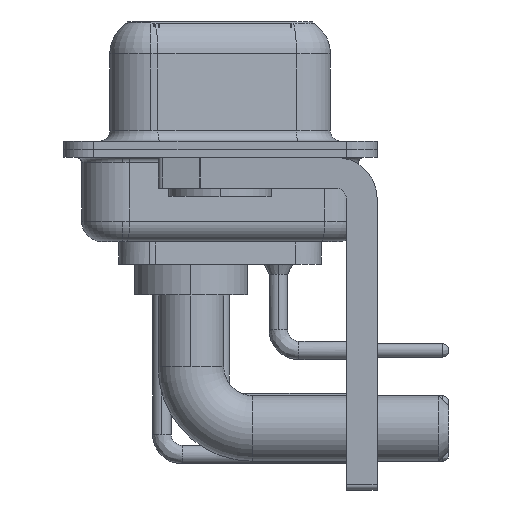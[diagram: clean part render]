
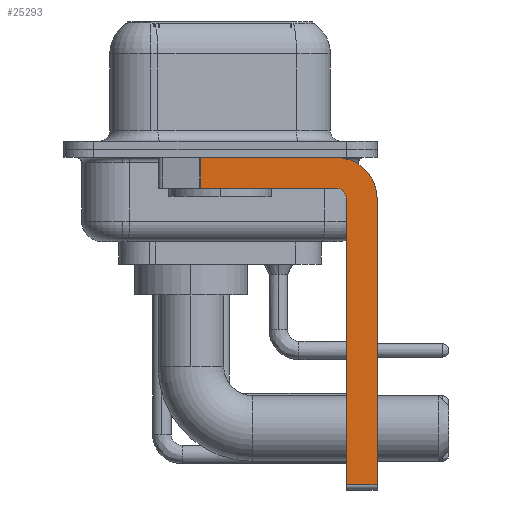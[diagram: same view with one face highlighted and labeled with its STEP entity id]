
A CAD part, left-side view. The second image highlights one B-rep face of the part: STEP entity #25293.
In plain terms, the highlighted planar face has unit normal (-1, 0, 0).
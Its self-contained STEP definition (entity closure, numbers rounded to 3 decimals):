
#324 = CARTESIAN_POINT ( 'NONE',  ( -2.9, -5.65, -16.35 ) ) ;
#525 = DIRECTION ( 'NONE',  ( 0., 0., 1. ) ) ;
#981 = CARTESIAN_POINT ( 'NONE',  ( -2.9, -7.65, -2.4 ) ) ;
#1199 = EDGE_CURVE ( 'NONE', #22641, #16061, #11977, .T. ) ;
#1399 = CIRCLE ( 'NONE', #16480, 0.5 ) ;
#1615 = CARTESIAN_POINT ( 'NONE',  ( -2.9, 0.978, -1.9 ) ) ;
#2493 = VERTEX_POINT ( 'NONE', #981 ) ;
#2877 = ORIENTED_EDGE ( 'NONE', *, *, #9466, .T. ) ;
#2976 = DIRECTION ( 'NONE',  ( 0., -1., 0. ) ) ;
#3555 = ORIENTED_EDGE ( 'NONE', *, *, #12667, .F. ) ;
#4824 = EDGE_CURVE ( 'NONE', #22641, #5567, #7491, .T. ) ;
#4982 = PLANE ( 'NONE',  #12929 ) ;
#5567 = VERTEX_POINT ( 'NONE', #6929 ) ;
#5573 = CARTESIAN_POINT ( 'NONE',  ( -2.9, -6.15, -16.6 ) ) ;
#6149 = CARTESIAN_POINT ( 'NONE',  ( -2.9, -5.65, -2.4 ) ) ;
#6283 = EDGE_CURVE ( 'NONE', #12804, #6546, #29942, .T. ) ;
#6546 = VERTEX_POINT ( 'NONE', #14704 ) ;
#6821 = CARTESIAN_POINT ( 'NONE',  ( -2.9, 3., -0.4 ) ) ;
#6929 = CARTESIAN_POINT ( 'NONE',  ( -2.9, -7.65, -16.35 ) ) ;
#7488 = VECTOR ( 'NONE', #13942, 1000. ) ;
#7491 = LINE ( 'NONE', #324, #19162 ) ;
#8713 = CARTESIAN_POINT ( 'NONE',  ( -2.9, -6.15, -2.4 ) ) ;
#8718 = VECTOR ( 'NONE', #23046, 1000. ) ;
#8973 = DIRECTION ( 'NONE',  ( 0., 0., 1. ) ) ;
#9212 = CARTESIAN_POINT ( 'NONE',  ( -2.9, -5.65, -1.9 ) ) ;
#9235 = LINE ( 'NONE', #11361, #7488 ) ;
#9466 = EDGE_CURVE ( 'NONE', #12804, #24037, #18348, .T. ) ;
#9821 = CARTESIAN_POINT ( 'NONE',  ( -2.9, 0.978, -0.4 ) ) ;
#10488 = EDGE_CURVE ( 'NONE', #16061, #29827, #1399, .T. ) ;
#11361 = CARTESIAN_POINT ( 'NONE',  ( -2.9, -7.65, -2.4 ) ) ;
#11977 = LINE ( 'NONE', #5573, #26487 ) ;
#12089 = VECTOR ( 'NONE', #13056, 1000. ) ;
#12667 = EDGE_CURVE ( 'NONE', #29827, #24037, #20325, .T. ) ;
#12804 = VERTEX_POINT ( 'NONE', #9821 ) ;
#12929 = AXIS2_PLACEMENT_3D ( 'NONE', #21411, #16991, #26300 ) ;
#13056 = DIRECTION ( 'NONE',  ( 0., 0., -1. ) ) ;
#13233 = EDGE_LOOP ( 'NONE', ( #20147, #2877, #3555, #13589, #25153, #18375, #18953, #22270 ) ) ;
#13294 = CARTESIAN_POINT ( 'NONE',  ( -2.9, 0.978, -1.9 ) ) ;
#13589 = ORIENTED_EDGE ( 'NONE', *, *, #10488, .F. ) ;
#13942 = DIRECTION ( 'NONE',  ( 0., 0., -1. ) ) ;
#14704 = CARTESIAN_POINT ( 'NONE',  ( -2.9, -5.65, -0.4 ) ) ;
#15478 = CARTESIAN_POINT ( 'NONE',  ( -2.9, -5.65, -1.9 ) ) ;
#16061 = VERTEX_POINT ( 'NONE', #8713 ) ;
#16480 = AXIS2_PLACEMENT_3D ( 'NONE', #6149, #18241, #8973 ) ;
#16564 = EDGE_CURVE ( 'NONE', #6546, #2493, #16664, .T. ) ;
#16664 = CIRCLE ( 'NONE', #26408, 2. ) ;
#16991 = DIRECTION ( 'NONE',  ( 1., 0., 0. ) ) ;
#17169 = EDGE_CURVE ( 'NONE', #2493, #5567, #9235, .T. ) ;
#17641 = DIRECTION ( 'NONE',  ( 0., 0., -1. ) ) ;
#18102 = CARTESIAN_POINT ( 'NONE',  ( -2.9, -6.15, -16.35 ) ) ;
#18194 = VECTOR ( 'NONE', #2976, 1000. ) ;
#18241 = DIRECTION ( 'NONE',  ( -1., 0., 0. ) ) ;
#18348 = LINE ( 'NONE', #1615, #12089 ) ;
#18375 = ORIENTED_EDGE ( 'NONE', *, *, #4824, .T. ) ;
#18901 = DIRECTION ( 'NONE',  ( 0., -1., 0. ) ) ;
#18953 = ORIENTED_EDGE ( 'NONE', *, *, #17169, .F. ) ;
#19162 = VECTOR ( 'NONE', #18901, 1000. ) ;
#20147 = ORIENTED_EDGE ( 'NONE', *, *, #6283, .F. ) ;
#20325 = LINE ( 'NONE', #9212, #8718 ) ;
#21263 = FACE_OUTER_BOUND ( 'NONE', #13233, .T. ) ;
#21411 = CARTESIAN_POINT ( 'NONE',  ( -2.9, -5.65, -2.4 ) ) ;
#22064 = DIRECTION ( 'NONE',  ( 1., 0., 0. ) ) ;
#22270 = ORIENTED_EDGE ( 'NONE', *, *, #16564, .F. ) ;
#22641 = VERTEX_POINT ( 'NONE', #18102 ) ;
#23046 = DIRECTION ( 'NONE',  ( 0., 1., 0. ) ) ;
#24037 = VERTEX_POINT ( 'NONE', #13294 ) ;
#24350 = CARTESIAN_POINT ( 'NONE',  ( -2.9, -5.65, -2.4 ) ) ;
#25153 = ORIENTED_EDGE ( 'NONE', *, *, #1199, .F. ) ;
#25293 = ADVANCED_FACE ( 'NONE', ( #21263 ), #4982, .F. ) ;
#26300 = DIRECTION ( 'NONE',  ( 0., 0., -1. ) ) ;
#26408 = AXIS2_PLACEMENT_3D ( 'NONE', #24350, #22064, #17641 ) ;
#26487 = VECTOR ( 'NONE', #525, 1000. ) ;
#29827 = VERTEX_POINT ( 'NONE', #15478 ) ;
#29942 = LINE ( 'NONE', #6821, #18194 ) ;
